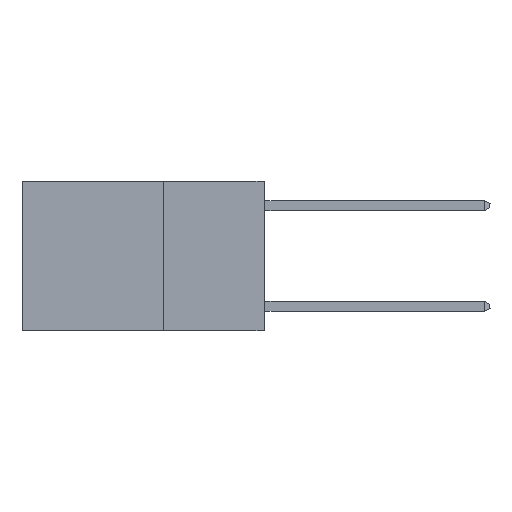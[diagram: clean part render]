
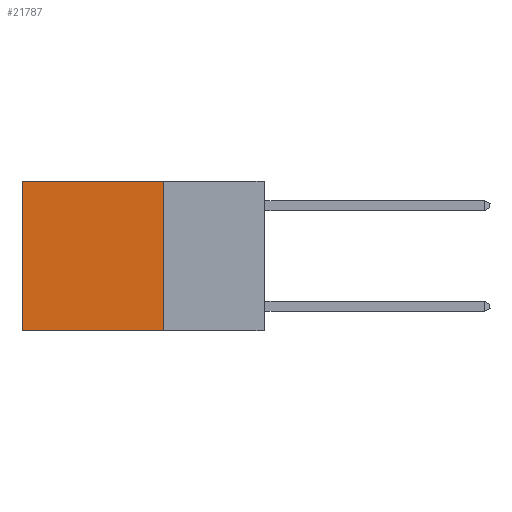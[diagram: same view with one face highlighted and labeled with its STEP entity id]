
A CAD part, left-side view. The second image highlights one B-rep face of the part: STEP entity #21787.
In plain terms, the highlighted planar face has unit normal (-1, 0, 0).
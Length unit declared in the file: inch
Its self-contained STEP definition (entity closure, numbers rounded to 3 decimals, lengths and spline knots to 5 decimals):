
#6 = DIRECTION ( 'NONE',  ( 0., 1., 0. ) ) ;
#37 = DIRECTION ( 'NONE',  ( 0., 1., 0. ) ) ;
#1513 = DIRECTION ( 'NONE',  ( 1., 0., 0. ) ) ;
#1933 = VERTEX_POINT ( 'NONE', #14492 ) ;
#3132 = EDGE_CURVE ( 'NONE', #19202, #21452, #23124, .T. ) ;
#3685 = VECTOR ( 'NONE', #4186, 39.37008 ) ;
#3726 = ORIENTED_EDGE ( 'NONE', *, *, #14847, .F. ) ;
#4186 = DIRECTION ( 'NONE',  ( 0., 0., -1. ) ) ;
#4662 = CARTESIAN_POINT ( 'NONE',  ( 0.2625, 0.6, 0. ) ) ;
#4788 = DIRECTION ( 'NONE',  ( 0., 0., -1. ) ) ;
#5233 = LINE ( 'NONE', #9206, #17586 ) ;
#7175 = FACE_OUTER_BOUND ( 'NONE', #11488, .T. ) ;
#7368 = CARTESIAN_POINT ( 'NONE',  ( 0.2625, 0.25, 0. ) ) ;
#9206 = CARTESIAN_POINT ( 'NONE',  ( 0.2625, 0.25, -0.37 ) ) ;
#9607 = CARTESIAN_POINT ( 'NONE',  ( 0.2625, 0.6, 0. ) ) ;
#9943 = ORIENTED_EDGE ( 'NONE', *, *, #3132, .T. ) ;
#10768 = ORIENTED_EDGE ( 'NONE', *, *, #21193, .F. ) ;
#11488 = EDGE_LOOP ( 'NONE', ( #9943, #3726, #10768, #17384 ) ) ;
#12381 = CARTESIAN_POINT ( 'NONE',  ( 0.2625, 0.25, 0. ) ) ;
#12591 = DIRECTION ( 'NONE',  ( 0., 0., -1. ) ) ;
#13263 = PLANE ( 'NONE',  #14126 ) ;
#13926 = EDGE_CURVE ( 'NONE', #1933, #19202, #16392, .T. ) ;
#14126 = AXIS2_PLACEMENT_3D ( 'NONE', #21590, #1513, #12591 ) ;
#14492 = CARTESIAN_POINT ( 'NONE',  ( 0.2625, 0.25, 0. ) ) ;
#14847 = EDGE_CURVE ( 'NONE', #17116, #21452, #5233, .T. ) ;
#15258 = VECTOR ( 'NONE', #4788, 39.37008 ) ;
#15263 = CARTESIAN_POINT ( 'NONE',  ( 0.2625, 0.6, -0.37 ) ) ;
#15693 = CARTESIAN_POINT ( 'NONE',  ( 0.2625, 0.25, -0.37 ) ) ;
#16392 = LINE ( 'NONE', #7368, #18915 ) ;
#17116 = VERTEX_POINT ( 'NONE', #15693 ) ;
#17384 = ORIENTED_EDGE ( 'NONE', *, *, #13926, .T. ) ;
#17586 = VECTOR ( 'NONE', #37, 39.37008 ) ;
#18915 = VECTOR ( 'NONE', #6, 39.37008 ) ;
#19202 = VERTEX_POINT ( 'NONE', #4662 ) ;
#19447 = LINE ( 'NONE', #12381, #15258 ) ;
#21193 = EDGE_CURVE ( 'NONE', #1933, #17116, #19447, .T. ) ;
#21452 = VERTEX_POINT ( 'NONE', #15263 ) ;
#21590 = CARTESIAN_POINT ( 'NONE',  ( 0.2625, 0.25, 0. ) ) ;
#21787 = ADVANCED_FACE ( 'NONE', ( #7175 ), #13263, .F. ) ;
#23124 = LINE ( 'NONE', #9607, #3685 ) ;
